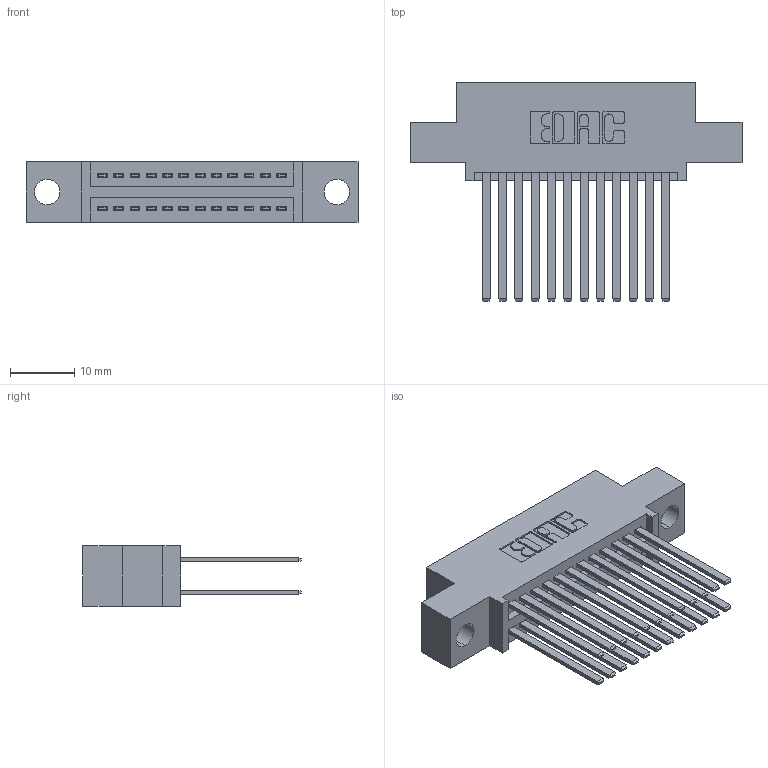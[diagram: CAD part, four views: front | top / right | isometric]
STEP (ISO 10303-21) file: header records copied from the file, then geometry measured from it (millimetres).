
FILE_DESCRIPTION (( 'STEP AP203' ), '1' );
FILE_NAME ('395-024-544-504.STEP', '2021-06-16T19:14:31', ( '' ), ( '' ), 'SwSTEP 2.0', 'SolidWorks 2020', '' );
FILE_SCHEMA (( 'CONFIG_CONTROL_DESIGN' ));
Length unit declared in the file: inch
Products named in the file (3): 345-292-001_345-293-144; 345 Part_0.110 Offset - 0.156 Dia-TI; 395-024-544-504
Assembly tree (25 placements, depth 2):
  395-024-544-504
    345 Part_0.110 Offset - 0.156 Dia-TI
    345-292-001_345-293-144  x24
Bounding box: 51.69 x 33.96 x 9.4 mm (x, y, z)
Volume: 4899.8 mm3; surface area: 7592.1 mm2
Topology: 25 solids, 25 shells, 1200 faces, 3533 edges, 2322 vertices
Faces by surface type: plane 794, cylinder 406
Entity records: 13821 total; most frequent: CARTESIAN_POINT 2350, ORIENTED_EDGE 2282, DIRECTION 2105, EDGE_CURVE 1141, VECTOR 965, LINE 965, VERTEX_POINT 758, AXIS2_PLACEMENT_3D 570
